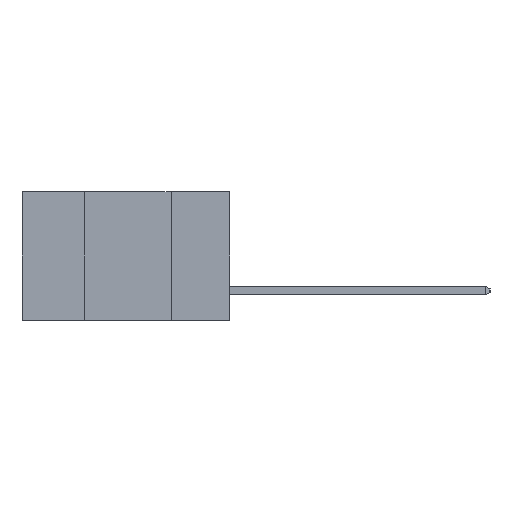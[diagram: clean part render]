
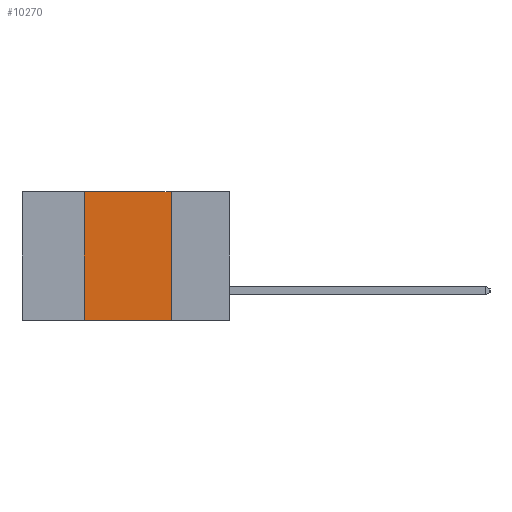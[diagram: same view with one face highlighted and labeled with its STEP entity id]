
A CAD part, left-side view. The second image highlights one B-rep face of the part: STEP entity #10270.
In plain terms, the highlighted planar face has unit normal (-1, 0, 0).
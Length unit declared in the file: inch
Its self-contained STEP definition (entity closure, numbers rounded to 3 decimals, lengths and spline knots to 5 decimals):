
#239 = ORIENTED_EDGE ( 'NONE', *, *, #3721, .F. ) ;
#560 = LINE ( 'NONE', #9643, #5282 ) ;
#860 = CARTESIAN_POINT ( 'NONE',  ( 0., 0.42, -0.37 ) ) ;
#1042 = LINE ( 'NONE', #10192, #7458 ) ;
#1597 = CARTESIAN_POINT ( 'NONE',  ( 0., 0.17, -0.37 ) ) ;
#2511 = VECTOR ( 'NONE', #9678, 39.37008 ) ;
#2688 = PLANE ( 'NONE',  #7321 ) ;
#2835 = DIRECTION ( 'NONE',  ( 0., 0., -1. ) ) ;
#3094 = CARTESIAN_POINT ( 'NONE',  ( 0., 0.17, 0. ) ) ;
#3721 = EDGE_CURVE ( 'NONE', #4883, #6511, #1042, .T. ) ;
#3724 = CARTESIAN_POINT ( 'NONE',  ( 0., 0.42, -0.37 ) ) ;
#3945 = EDGE_CURVE ( 'NONE', #5162, #4883, #9647, .T. ) ;
#4883 = VERTEX_POINT ( 'NONE', #4936 ) ;
#4936 = CARTESIAN_POINT ( 'NONE',  ( 0., 0.42, 0. ) ) ;
#5162 = VERTEX_POINT ( 'NONE', #860 ) ;
#5219 = VECTOR ( 'NONE', #8815, 39.37008 ) ;
#5257 = ORIENTED_EDGE ( 'NONE', *, *, #3945, .F. ) ;
#5282 = VECTOR ( 'NONE', #2835, 39.37008 ) ;
#5359 = DIRECTION ( 'NONE',  ( 0., 0., -1. ) ) ;
#5553 = CARTESIAN_POINT ( 'NONE',  ( 0., 0.6, -0.37 ) ) ;
#6511 = VERTEX_POINT ( 'NONE', #3094 ) ;
#6998 = EDGE_LOOP ( 'NONE', ( #8404, #239, #5257, #7512 ) ) ;
#7017 = CARTESIAN_POINT ( 'NONE',  ( 0., 0.6, 0. ) ) ;
#7321 = AXIS2_PLACEMENT_3D ( 'NONE', #7017, #10336, #5359 ) ;
#7458 = VECTOR ( 'NONE', #9364, 39.37008 ) ;
#7495 = FACE_OUTER_BOUND ( 'NONE', #6998, .T. ) ;
#7512 = ORIENTED_EDGE ( 'NONE', *, *, #7539, .T. ) ;
#7539 = EDGE_CURVE ( 'NONE', #5162, #10139, #9315, .T. ) ;
#8404 = ORIENTED_EDGE ( 'NONE', *, *, #8599, .F. ) ;
#8599 = EDGE_CURVE ( 'NONE', #6511, #10139, #560, .T. ) ;
#8815 = DIRECTION ( 'NONE',  ( 0., 0., 1. ) ) ;
#9315 = LINE ( 'NONE', #5553, #2511 ) ;
#9364 = DIRECTION ( 'NONE',  ( 0., -1., 0. ) ) ;
#9643 = CARTESIAN_POINT ( 'NONE',  ( 0., 0.17, -0.37 ) ) ;
#9647 = LINE ( 'NONE', #3724, #5219 ) ;
#9678 = DIRECTION ( 'NONE',  ( 0., -1., 0. ) ) ;
#10139 = VERTEX_POINT ( 'NONE', #1597 ) ;
#10192 = CARTESIAN_POINT ( 'NONE',  ( 0., 0.6, 0. ) ) ;
#10270 = ADVANCED_FACE ( 'NONE', ( #7495 ), #2688, .F. ) ;
#10336 = DIRECTION ( 'NONE',  ( 1., 0., 0. ) ) ;
